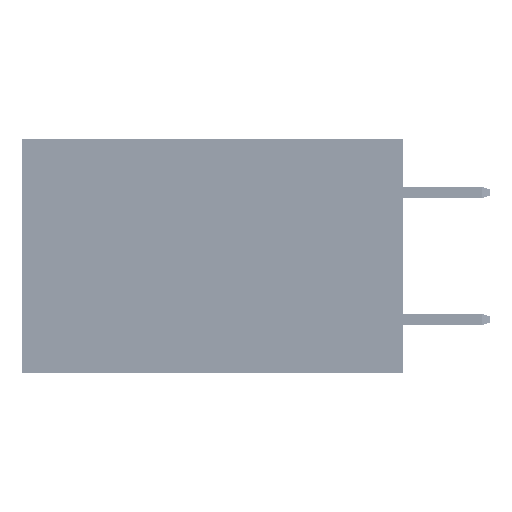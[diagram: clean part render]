
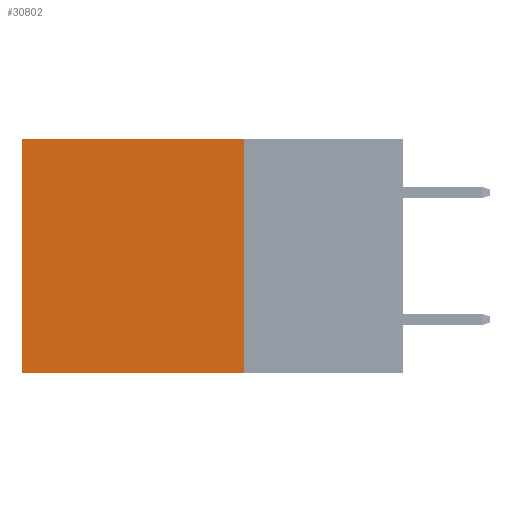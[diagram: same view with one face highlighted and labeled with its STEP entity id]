
A CAD part, left-side view. The second image highlights one B-rep face of the part: STEP entity #30802.
In plain terms, the highlighted planar face has unit normal (-1, 0, 0).
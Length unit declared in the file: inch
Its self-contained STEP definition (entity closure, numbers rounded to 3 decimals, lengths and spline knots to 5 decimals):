
#98 = EDGE_CURVE ( 'NONE', #16003, #13171, #28480, .T. ) ;
#1632 = AXIS2_PLACEMENT_3D ( 'NONE', #13990, #43978, #10331 ) ;
#5642 = LINE ( 'NONE', #42516, #8025 ) ;
#6022 = CARTESIAN_POINT ( 'NONE',  ( 0.2875, 0.25, 0. ) ) ;
#6032 = LINE ( 'NONE', #32332, #40877 ) ;
#7737 = CARTESIAN_POINT ( 'NONE',  ( 0.2875, 0.6, -0.37 ) ) ;
#8025 = VECTOR ( 'NONE', #39051, 39.37008 ) ;
#9816 = VERTEX_POINT ( 'NONE', #28437 ) ;
#10025 = LINE ( 'NONE', #28443, #24557 ) ;
#10331 = DIRECTION ( 'NONE',  ( 0., 0., -1. ) ) ;
#11277 = EDGE_CURVE ( 'NONE', #9816, #13171, #10025, .T. ) ;
#13171 = VERTEX_POINT ( 'NONE', #7737 ) ;
#13990 = CARTESIAN_POINT ( 'NONE',  ( 0.2875, 0.25, 0. ) ) ;
#16003 = VERTEX_POINT ( 'NONE', #19972 ) ;
#16076 = EDGE_LOOP ( 'NONE', ( #42838, #24845, #48410, #26299 ) ) ;
#19972 = CARTESIAN_POINT ( 'NONE',  ( 0.2875, 0.25, -0.37 ) ) ;
#24557 = VECTOR ( 'NONE', #28685, 39.37008 ) ;
#24778 = CARTESIAN_POINT ( 'NONE',  ( 0.2875, 0.25, -0.37 ) ) ;
#24845 = ORIENTED_EDGE ( 'NONE', *, *, #98, .F. ) ;
#26299 = ORIENTED_EDGE ( 'NONE', *, *, #42618, .T. ) ;
#26542 = VERTEX_POINT ( 'NONE', #6022 ) ;
#28437 = CARTESIAN_POINT ( 'NONE',  ( 0.2875, 0.6, 0. ) ) ;
#28443 = CARTESIAN_POINT ( 'NONE',  ( 0.2875, 0.6, 0. ) ) ;
#28480 = LINE ( 'NONE', #24778, #32687 ) ;
#28685 = DIRECTION ( 'NONE',  ( 0., 0., -1. ) ) ;
#29234 = FACE_OUTER_BOUND ( 'NONE', #16076, .T. ) ;
#30802 = ADVANCED_FACE ( 'NONE', ( #29234 ), #47659, .F. ) ;
#31598 = DIRECTION ( 'NONE',  ( 0., 0., -1. ) ) ;
#32332 = CARTESIAN_POINT ( 'NONE',  ( 0.2875, 0.25, 0. ) ) ;
#32557 = EDGE_CURVE ( 'NONE', #26542, #16003, #6032, .T. ) ;
#32687 = VECTOR ( 'NONE', #39764, 39.37008 ) ;
#39051 = DIRECTION ( 'NONE',  ( 0., 1., 0. ) ) ;
#39764 = DIRECTION ( 'NONE',  ( 0., 1., 0. ) ) ;
#40877 = VECTOR ( 'NONE', #31598, 39.37008 ) ;
#42516 = CARTESIAN_POINT ( 'NONE',  ( 0.2875, 0.25, 0. ) ) ;
#42618 = EDGE_CURVE ( 'NONE', #26542, #9816, #5642, .T. ) ;
#42838 = ORIENTED_EDGE ( 'NONE', *, *, #11277, .T. ) ;
#43978 = DIRECTION ( 'NONE',  ( 1., 0., 0. ) ) ;
#47659 = PLANE ( 'NONE',  #1632 ) ;
#48410 = ORIENTED_EDGE ( 'NONE', *, *, #32557, .F. ) ;
